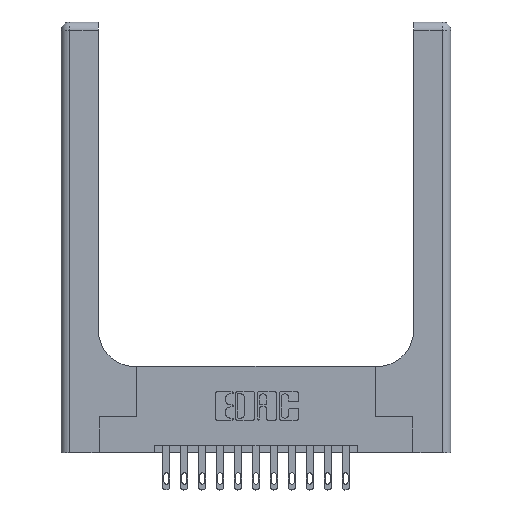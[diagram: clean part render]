
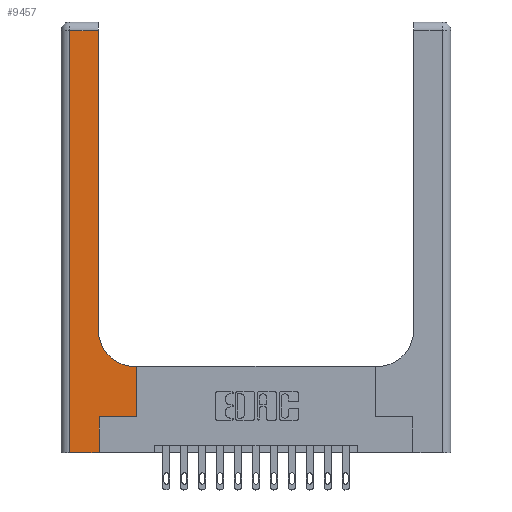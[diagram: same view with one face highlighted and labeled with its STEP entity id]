
A CAD part, top view. The second image highlights one B-rep face of the part: STEP entity #9457.
In plain terms, the highlighted planar face has unit normal (0, 0, 1).
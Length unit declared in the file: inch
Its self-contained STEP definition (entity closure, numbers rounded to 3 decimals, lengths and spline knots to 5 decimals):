
#17 = LINE ( 'NONE', #7868, #9022 ) ;
#126 = CARTESIAN_POINT ( 'NONE',  ( 0.26, 2.94, 0.37 ) ) ;
#161 = VERTEX_POINT ( 'NONE', #15169 ) ;
#315 = AXIS2_PLACEMENT_3D ( 'NONE', #11417, #8288, #5544 ) ;
#447 = EDGE_CURVE ( 'NONE', #3765, #14213, #681, .T. ) ;
#630 = CARTESIAN_POINT ( 'NONE',  ( 0., 2.94, 0.37 ) ) ;
#681 = LINE ( 'NONE', #1647, #6796 ) ;
#754 = VERTEX_POINT ( 'NONE', #10193 ) ;
#781 = EDGE_CURVE ( 'NONE', #8550, #754, #3681, .T. ) ;
#873 = CARTESIAN_POINT ( 'NONE',  ( 0.26, 3., 0.37 ) ) ;
#1018 = DIRECTION ( 'NONE',  ( 1., 0., 0. ) ) ;
#1281 = ORIENTED_EDGE ( 'NONE', *, *, #4845, .T. ) ;
#1296 = DIRECTION ( 'NONE',  ( 0., 0., -1. ) ) ;
#1398 = VERTEX_POINT ( 'NONE', #9472 ) ;
#1647 = CARTESIAN_POINT ( 'NONE',  ( 0.265, 0., 0.37 ) ) ;
#2076 = EDGE_CURVE ( 'NONE', #8784, #1398, #14671, .T. ) ;
#2094 = DIRECTION ( 'NONE',  ( 0., -1., 0. ) ) ;
#2614 = CARTESIAN_POINT ( 'NONE',  ( 0.265, 0.25, 0.37 ) ) ;
#2819 = CIRCLE ( 'NONE', #11819, 0.25 ) ;
#2907 = DIRECTION ( 'NONE',  ( 0., 1., 0. ) ) ;
#3681 = LINE ( 'NONE', #14126, #12281 ) ;
#3765 = VERTEX_POINT ( 'NONE', #12038 ) ;
#3923 = EDGE_CURVE ( 'NONE', #12183, #3765, #6106, .T. ) ;
#4730 = DIRECTION ( 'NONE',  ( 0., 1., 0. ) ) ;
#4845 = EDGE_CURVE ( 'NONE', #14213, #161, #17, .T. ) ;
#4933 = DIRECTION ( 'NONE',  ( 0., 1., 0. ) ) ;
#5040 = DIRECTION ( 'NONE',  ( -1., 0., 0. ) ) ;
#5544 = DIRECTION ( 'NONE',  ( -1., 0., 0. ) ) ;
#5925 = VECTOR ( 'NONE', #4730, 39.37008 ) ;
#6106 = LINE ( 'NONE', #7760, #14232 ) ;
#6183 = PLANE ( 'NONE',  #315 ) ;
#6193 = DIRECTION ( 'NONE',  ( 1., 0., 0. ) ) ;
#6220 = EDGE_CURVE ( 'NONE', #15255, #8784, #16508, .T. ) ;
#6319 = ORIENTED_EDGE ( 'NONE', *, *, #12160, .T. ) ;
#6796 = VECTOR ( 'NONE', #2907, 39.37008 ) ;
#6980 = EDGE_CURVE ( 'NONE', #161, #8550, #7555, .T. ) ;
#7220 = CARTESIAN_POINT ( 'NONE',  ( 0.528, 0.25, 0.37 ) ) ;
#7285 = CARTESIAN_POINT ( 'NONE',  ( 0.528, 0.6, 0.37 ) ) ;
#7492 = FACE_OUTER_BOUND ( 'NONE', #11156, .T. ) ;
#7555 = LINE ( 'NONE', #7220, #5925 ) ;
#7655 = ORIENTED_EDGE ( 'NONE', *, *, #6980, .T. ) ;
#7760 = CARTESIAN_POINT ( 'NONE',  ( 0., 0., 0.37 ) ) ;
#7868 = CARTESIAN_POINT ( 'NONE',  ( 0.265, 0.25, 0.37 ) ) ;
#8288 = DIRECTION ( 'NONE',  ( 0., 0., -1. ) ) ;
#8550 = VERTEX_POINT ( 'NONE', #7285 ) ;
#8784 = VERTEX_POINT ( 'NONE', #126 ) ;
#9022 = VECTOR ( 'NONE', #14557, 39.37008 ) ;
#9146 = CARTESIAN_POINT ( 'NONE',  ( 0.51, 0.85, 0.37 ) ) ;
#9218 = VECTOR ( 'NONE', #13304, 39.37008 ) ;
#9457 = ADVANCED_FACE ( 'NONE', ( #7492 ), #6183, .F. ) ;
#9472 = CARTESIAN_POINT ( 'NONE',  ( 0.06, 2.94, 0.37 ) ) ;
#9606 = CARTESIAN_POINT ( 'NONE',  ( 0.06, 0., 0.37 ) ) ;
#9613 = ORIENTED_EDGE ( 'NONE', *, *, #6220, .T. ) ;
#9800 = CARTESIAN_POINT ( 'NONE',  ( 0.26, 0.85, 0.37 ) ) ;
#10193 = CARTESIAN_POINT ( 'NONE',  ( 0.51, 0.6, 0.37 ) ) ;
#10264 = ORIENTED_EDGE ( 'NONE', *, *, #11018, .T. ) ;
#11018 = EDGE_CURVE ( 'NONE', #754, #15255, #2819, .T. ) ;
#11156 = EDGE_LOOP ( 'NONE', ( #9613, #14178, #6319, #15189, #14773, #1281, #7655, #15395, #10264 ) ) ;
#11277 = VECTOR ( 'NONE', #2094, 39.37008 ) ;
#11417 = CARTESIAN_POINT ( 'NONE',  ( 0., 3., 0.37 ) ) ;
#11819 = AXIS2_PLACEMENT_3D ( 'NONE', #9146, #1296, #6193 ) ;
#12038 = CARTESIAN_POINT ( 'NONE',  ( 0.265, 0., 0.37 ) ) ;
#12055 = VECTOR ( 'NONE', #4933, 39.37008 ) ;
#12160 = EDGE_CURVE ( 'NONE', #1398, #12183, #12319, .T. ) ;
#12183 = VERTEX_POINT ( 'NONE', #9606 ) ;
#12281 = VECTOR ( 'NONE', #5040, 39.37008 ) ;
#12319 = LINE ( 'NONE', #13703, #11277 ) ;
#13304 = DIRECTION ( 'NONE',  ( -1., 0., 0. ) ) ;
#13703 = CARTESIAN_POINT ( 'NONE',  ( 0.06, 3., 0.37 ) ) ;
#14126 = CARTESIAN_POINT ( 'NONE',  ( 0.26, 0.6, 0.37 ) ) ;
#14178 = ORIENTED_EDGE ( 'NONE', *, *, #2076, .T. ) ;
#14213 = VERTEX_POINT ( 'NONE', #2614 ) ;
#14232 = VECTOR ( 'NONE', #1018, 39.37008 ) ;
#14557 = DIRECTION ( 'NONE',  ( 1., 0., 0. ) ) ;
#14671 = LINE ( 'NONE', #630, #9218 ) ;
#14773 = ORIENTED_EDGE ( 'NONE', *, *, #447, .T. ) ;
#15169 = CARTESIAN_POINT ( 'NONE',  ( 0.528, 0.25, 0.37 ) ) ;
#15189 = ORIENTED_EDGE ( 'NONE', *, *, #3923, .T. ) ;
#15255 = VERTEX_POINT ( 'NONE', #9800 ) ;
#15395 = ORIENTED_EDGE ( 'NONE', *, *, #781, .T. ) ;
#16508 = LINE ( 'NONE', #873, #12055 ) ;
